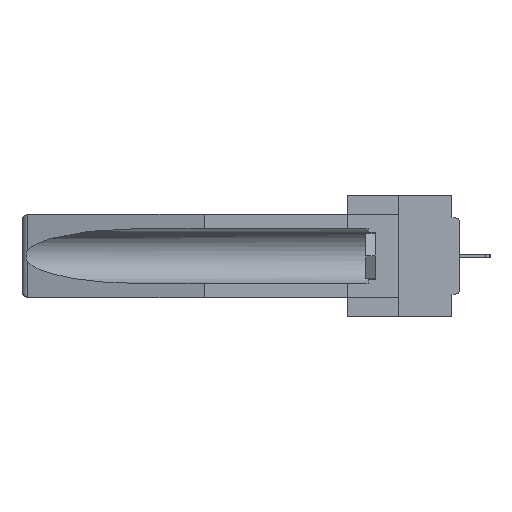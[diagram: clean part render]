
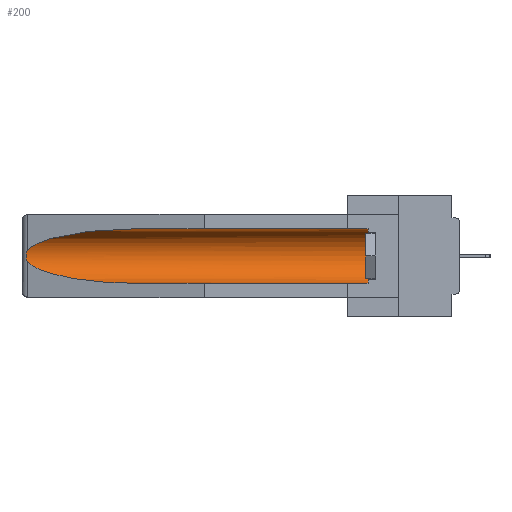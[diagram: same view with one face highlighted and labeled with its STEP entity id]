
A CAD part, left-side view. The second image highlights one B-rep face of the part: STEP entity #200.
In plain terms, the highlighted cylindrical face has radius 2.857 mm (diameter 5.715 mm), a partial arc.
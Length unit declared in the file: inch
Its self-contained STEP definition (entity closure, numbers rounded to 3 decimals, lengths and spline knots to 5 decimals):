
#50 = CARTESIAN_POINT ( 'NONE',  ( 0.26537, 1.52718, -0.14972 ) ) ;
#91 = CARTESIAN_POINT ( 'NONE',  ( 0.155, 0.126, -0.059 ) ) ;
#158 = CARTESIAN_POINT ( 'NONE',  ( 0.26597, 1.5296, -0.19026 ) ) ;
#200 = ADVANCED_FACE ( 'NONE', ( #28317 ), #14190, .F. ) ;
#1684 =( BOUNDED_CURVE ( )  B_SPLINE_CURVE ( 3, ( #11100, #26167, #8520, #13629 ),
 .UNSPECIFIED., .F., .F. ) 
 B_SPLINE_CURVE_WITH_KNOTS ( ( 4, 4 ),
 ( 0.1948, 1.5708 ),
 .UNSPECIFIED. ) 
 CURVE ( )  GEOMETRIC_REPRESENTATION_ITEM ( )  RATIONAL_B_SPLINE_CURVE ( ( 1., 0.848, 0.848, 1. ) ) 
 REPRESENTATION_ITEM ( '' )  );
#2689 = CARTESIAN_POINT ( 'NONE',  ( 0.26597, 1.52961, -0.15275 ) ) ;
#3646 = EDGE_LOOP ( 'NONE', ( #8231, #15532, #9490, #14052, #14902, #6302 ) ) ;
#4081 = CARTESIAN_POINT ( 'NONE',  ( 0.25451, 1.48313, -0.09465 ) ) ;
#5274 = CARTESIAN_POINT ( 'NONE',  ( 0.155, -0.30754, -0.1715 ) ) ;
#5545 = DIRECTION ( 'NONE',  ( 0., 0., 1. ) ) ;
#6144 = AXIS2_PLACEMENT_3D ( 'NONE', #9371, #26991, #11931 ) ;
#6302 = ORIENTED_EDGE ( 'NONE', *, *, #13022, .T. ) ;
#7308 = VECTOR ( 'NONE', #16803, 39.37008 ) ;
#7772 = CARTESIAN_POINT ( 'NONE',  ( 0.155, 1.07973, -0.284 ) ) ;
#8012 = EDGE_CURVE ( 'NONE', #12752, #26647, #1684, .T. ) ;
#8231 = ORIENTED_EDGE ( 'NONE', *, *, #12287, .T. ) ;
#8279 = LINE ( 'NONE', #12653, #28361 ) ;
#8520 = CARTESIAN_POINT ( 'NONE',  ( 0.21114, 1.30732, -0.284 ) ) ;
#9141 = CARTESIAN_POINT ( 'NONE',  ( 0.155, -0.30754, -0.284 ) ) ;
#9371 = CARTESIAN_POINT ( 'NONE',  ( 0.155, 0.126, -0.1715 ) ) ;
#9490 = ORIENTED_EDGE ( 'NONE', *, *, #8012, .T. ) ;
#10443 = CARTESIAN_POINT ( 'NONE',  ( 0.2673, 1.5327, -0.16383 ) ) ;
#11068 = EDGE_CURVE ( 'NONE', #13309, #12752, #29211, .T. ) ;
#11100 = CARTESIAN_POINT ( 'NONE',  ( 0.26537, 1.52718, -0.19328 ) ) ;
#11786 = CARTESIAN_POINT ( 'NONE',  ( 0.155, 1.07973, -0.059 ) ) ;
#11931 = DIRECTION ( 'NONE',  ( 0., 0., 1. ) ) ;
#12287 = EDGE_CURVE ( 'NONE', #16565, #13309, #28309, .T. ) ;
#12548 = DIRECTION ( 'NONE',  ( 0., 1., 0. ) ) ;
#12653 = CARTESIAN_POINT ( 'NONE',  ( 0.155, -0.30754, -0.059 ) ) ;
#12752 = VERTEX_POINT ( 'NONE', #21753 ) ;
#12974 = CARTESIAN_POINT ( 'NONE',  ( 0.2675, 1.53308, -0.17534 ) ) ;
#13022 = EDGE_CURVE ( 'NONE', #31080, #16565, #8279, .T. ) ;
#13291 = CIRCLE ( 'NONE', #6144, 0.1125 ) ;
#13309 = VERTEX_POINT ( 'NONE', #28769 ) ;
#13629 = CARTESIAN_POINT ( 'NONE',  ( 0.155, 1.07973, -0.284 ) ) ;
#13906 = CARTESIAN_POINT ( 'NONE',  ( 0.155, 0.126, -0.284 ) ) ;
#14052 = ORIENTED_EDGE ( 'NONE', *, *, #15927, .F. ) ;
#14087 = LINE ( 'NONE', #9141, #7308 ) ;
#14190 = CYLINDRICAL_SURFACE ( 'NONE', #20384, 0.1125 ) ;
#14240 = CARTESIAN_POINT ( 'NONE',  ( 0.155, 1.07973, -0.059 ) ) ;
#14902 = ORIENTED_EDGE ( 'NONE', *, *, #15965, .T. ) ;
#15532 = ORIENTED_EDGE ( 'NONE', *, *, #11068, .T. ) ;
#15543 = CARTESIAN_POINT ( 'NONE',  ( 0.26655, 1.53094, -0.18657 ) ) ;
#15927 = EDGE_CURVE ( 'NONE', #21760, #26647, #14087, .T. ) ;
#15965 = EDGE_CURVE ( 'NONE', #21760, #31080, #13291, .T. ) ;
#16565 = VERTEX_POINT ( 'NONE', #11786 ) ;
#16803 = DIRECTION ( 'NONE',  ( 0., 1., 0. ) ) ;
#18069 = CARTESIAN_POINT ( 'NONE',  ( 0.26537, 1.52718, -0.19328 ) ) ;
#20384 = AXIS2_PLACEMENT_3D ( 'NONE', #5274, #31275, #5545 ) ;
#21753 = CARTESIAN_POINT ( 'NONE',  ( 0.26537, 1.52718, -0.19328 ) ) ;
#21760 = VERTEX_POINT ( 'NONE', #13906 ) ;
#21885 = CARTESIAN_POINT ( 'NONE',  ( 0.26537, 1.52718, -0.14972 ) ) ;
#25538 = CARTESIAN_POINT ( 'NONE',  ( 0.26654, 1.53092, -0.15636 ) ) ;
#26167 = CARTESIAN_POINT ( 'NONE',  ( 0.25451, 1.48313, -0.24835 ) ) ;
#26647 = VERTEX_POINT ( 'NONE', #7772 ) ;
#26779 = CARTESIAN_POINT ( 'NONE',  ( 0.21114, 1.30732, -0.059 ) ) ;
#26991 = DIRECTION ( 'NONE',  ( 0., -1., 0. ) ) ;
#28027 = CARTESIAN_POINT ( 'NONE',  ( 0.2675, 1.53308, -0.16763 ) ) ;
#28309 =( BOUNDED_CURVE ( )  B_SPLINE_CURVE ( 3, ( #14240, #26779, #4081, #21885 ),
 .UNSPECIFIED., .F., .T. ) 
 B_SPLINE_CURVE_WITH_KNOTS ( ( 4, 4 ),
 ( 4.71239, 6.08839 ),
 .UNSPECIFIED. ) 
 CURVE ( )  GEOMETRIC_REPRESENTATION_ITEM ( )  RATIONAL_B_SPLINE_CURVE ( ( 1., 0.848, 0.848, 1. ) ) 
 REPRESENTATION_ITEM ( '' )  );
#28317 = FACE_OUTER_BOUND ( 'NONE', #3646, .T. ) ;
#28361 = VECTOR ( 'NONE', #12548, 39.37008 ) ;
#28769 = CARTESIAN_POINT ( 'NONE',  ( 0.26537, 1.52718, -0.14972 ) ) ;
#29211 = B_SPLINE_CURVE_WITH_KNOTS ( 'NONE', 3,
 ( #50, #2689, #25538, #10443, #28027, #12974, #30495, #15543, #158, #18069 ),
 .UNSPECIFIED., .F., .F.,
 ( 4, 2, 2, 2, 4 ),
 ( 0., 0.00029, 0.00058, 0.00087, 0.00117 ),
 .UNSPECIFIED. ) ;
#30495 = CARTESIAN_POINT ( 'NONE',  ( 0.2673, 1.53269, -0.17917 ) ) ;
#31080 = VERTEX_POINT ( 'NONE', #91 ) ;
#31275 = DIRECTION ( 'NONE',  ( 0., 1., 0. ) ) ;
